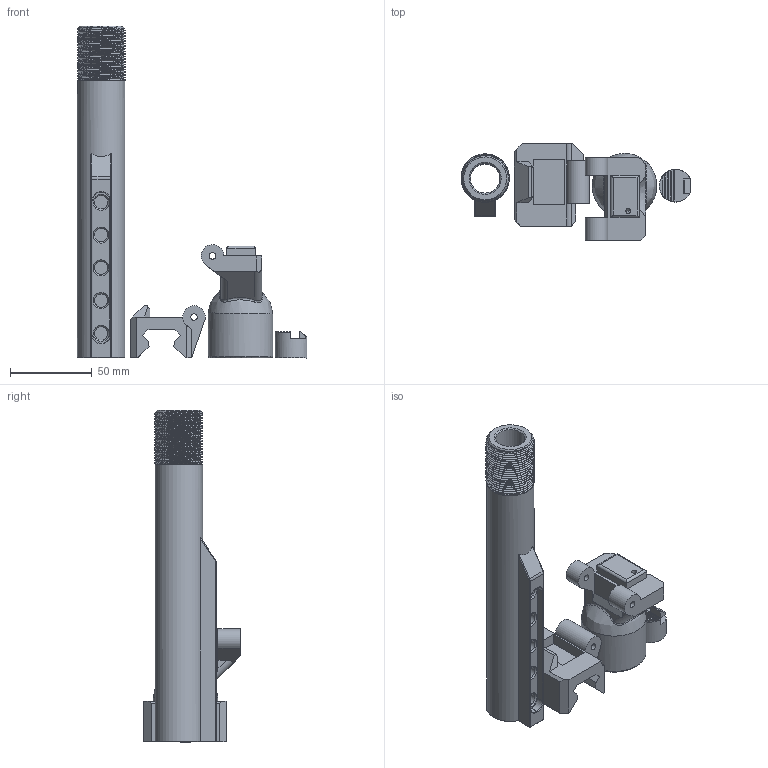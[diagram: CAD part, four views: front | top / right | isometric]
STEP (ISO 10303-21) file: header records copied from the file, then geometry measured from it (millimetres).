
FILE_DESCRIPTION(/* description */ (''),/* implementation_level */ '2;1');
FILE_NAME(/* author */ (''),/* organization */ (''),/* preprocessor_version */ 'ST-DEVELOPER v15.2',/* originating_system */ 'Autodesk Translator Framework v2.0.0.5431',/* authorisation */ '');
FILE_SCHEMA (('AUTOMOTIVE_DESIGN { 1 0 10303 214 3 1 1 }'));
Length unit declared in the file: centimetre
Products named in the file (1): unpublished stocks
Bounding box: 140.23 x 59.1 x 202.53 mm (x, y, z)
Volume: 170255.2 mm3; surface area: 67103.5 mm2
Topology: 4 solids, 4 shells, 257 faces, 772 edges, 531 vertices
Faces by surface type: plane 134, cylinder 57, bspline 43, cone 16, torus 7
Full cylindrical faces by diameter (mm): 3 x1, 4 x3, 8.2 x5, 12.1 x1, 18 x1, 20.5 x1, 29 x1, 30.8 x1, 39.4 x1
Entity records: 28377 total; most frequent: CARTESIAN_POINT 21997, ORIENTED_EDGE 1454, DIRECTION 1130, EDGE_CURVE 727, VERTEX_POINT 515, AXIS2_PLACEMENT_3D 405, LINE 320, VECTOR 320
